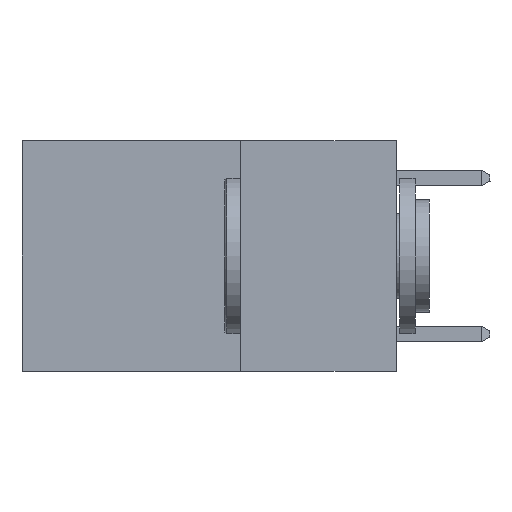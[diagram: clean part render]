
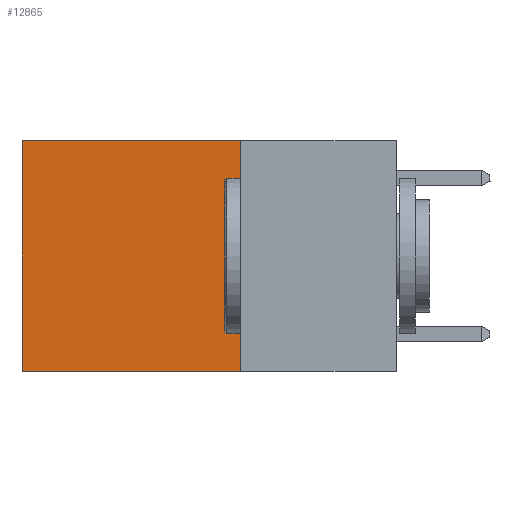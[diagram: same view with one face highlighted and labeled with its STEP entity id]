
A CAD part, left-side view. The second image highlights one B-rep face of the part: STEP entity #12865.
In plain terms, the highlighted planar face has unit normal (-1, 0, 0).
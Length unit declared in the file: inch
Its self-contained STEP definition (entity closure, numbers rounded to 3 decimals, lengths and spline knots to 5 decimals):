
#664 = VECTOR ( 'NONE', #22723, 39.37008 ) ;
#760 = DIRECTION ( 'NONE',  ( 0., 1., 0. ) ) ;
#1501 = VECTOR ( 'NONE', #14976, 39.37008 ) ;
#1853 = CARTESIAN_POINT ( 'NONE',  ( 0.2625, 0.25, 0. ) ) ;
#2208 = ORIENTED_EDGE ( 'NONE', *, *, #15385, .F. ) ;
#3301 = AXIS2_PLACEMENT_3D ( 'NONE', #1853, #25648, #4067 ) ;
#4067 = DIRECTION ( 'NONE',  ( 0., 0., -1. ) ) ;
#4217 = FACE_OUTER_BOUND ( 'NONE', #23984, .T. ) ;
#4348 = EDGE_CURVE ( 'NONE', #4753, #26183, #25167, .T. ) ;
#4753 = VERTEX_POINT ( 'NONE', #6197 ) ;
#5020 = VERTEX_POINT ( 'NONE', #9797 ) ;
#5057 = LINE ( 'NONE', #14654, #1501 ) ;
#6197 = CARTESIAN_POINT ( 'NONE',  ( 0.2625, 0.25, -0.37 ) ) ;
#6203 = VECTOR ( 'NONE', #760, 39.37008 ) ;
#6529 = CARTESIAN_POINT ( 'NONE',  ( 0.2625, 0.6, 0. ) ) ;
#8474 = CARTESIAN_POINT ( 'NONE',  ( 0.2625, 0.25, 0. ) ) ;
#9117 = PLANE ( 'NONE',  #3301 ) ;
#9797 = CARTESIAN_POINT ( 'NONE',  ( 0.2625, 0.6, 0. ) ) ;
#9878 = VECTOR ( 'NONE', #17058, 39.37008 ) ;
#10892 = EDGE_CURVE ( 'NONE', #5020, #26183, #20975, .T. ) ;
#12602 = CARTESIAN_POINT ( 'NONE',  ( 0.2625, 0.25, -0.37 ) ) ;
#12865 = ADVANCED_FACE ( 'NONE', ( #4217 ), #9117, .F. ) ;
#13368 = ORIENTED_EDGE ( 'NONE', *, *, #10892, .T. ) ;
#14654 = CARTESIAN_POINT ( 'NONE',  ( 0.2625, 0.25, 0. ) ) ;
#14976 = DIRECTION ( 'NONE',  ( 0., 1., 0. ) ) ;
#15385 = EDGE_CURVE ( 'NONE', #19282, #4753, #16737, .T. ) ;
#16737 = LINE ( 'NONE', #23656, #9878 ) ;
#17058 = DIRECTION ( 'NONE',  ( 0., 0., -1. ) ) ;
#19282 = VERTEX_POINT ( 'NONE', #8474 ) ;
#20163 = CARTESIAN_POINT ( 'NONE',  ( 0.2625, 0.6, -0.37 ) ) ;
#20975 = LINE ( 'NONE', #6529, #664 ) ;
#22071 = ORIENTED_EDGE ( 'NONE', *, *, #22125, .T. ) ;
#22125 = EDGE_CURVE ( 'NONE', #19282, #5020, #5057, .T. ) ;
#22723 = DIRECTION ( 'NONE',  ( 0., 0., -1. ) ) ;
#23656 = CARTESIAN_POINT ( 'NONE',  ( 0.2625, 0.25, 0. ) ) ;
#23984 = EDGE_LOOP ( 'NONE', ( #13368, #25263, #2208, #22071 ) ) ;
#25167 = LINE ( 'NONE', #12602, #6203 ) ;
#25263 = ORIENTED_EDGE ( 'NONE', *, *, #4348, .F. ) ;
#25648 = DIRECTION ( 'NONE',  ( 1., 0., 0. ) ) ;
#26183 = VERTEX_POINT ( 'NONE', #20163 ) ;
